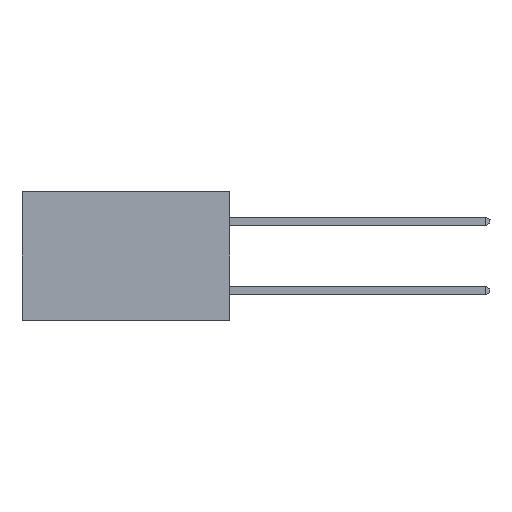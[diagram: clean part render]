
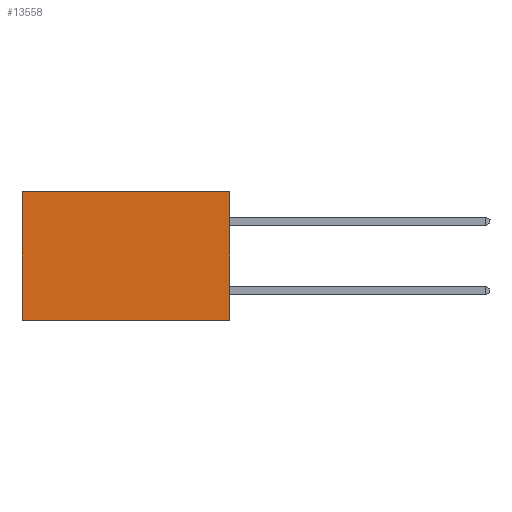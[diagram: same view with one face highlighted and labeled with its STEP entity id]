
A CAD part, left-side view. The second image highlights one B-rep face of the part: STEP entity #13558.
In plain terms, the highlighted planar face has unit normal (-1, 0, 0).
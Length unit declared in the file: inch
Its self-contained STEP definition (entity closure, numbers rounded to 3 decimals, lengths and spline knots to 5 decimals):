
#208 = EDGE_CURVE ( 'NONE', #3559, #17901, #7418, .T. ) ;
#286 = AXIS2_PLACEMENT_3D ( 'NONE', #8222, #3590, #12796 ) ;
#575 = VERTEX_POINT ( 'NONE', #19962 ) ;
#1164 = PLANE ( 'NONE',  #286 ) ;
#3559 = VERTEX_POINT ( 'NONE', #4730 ) ;
#3590 = DIRECTION ( 'NONE',  ( 1., 0., 0. ) ) ;
#4028 = CARTESIAN_POINT ( 'NONE',  ( 0.298, 0., -0.37 ) ) ;
#4073 = EDGE_CURVE ( 'NONE', #17901, #575, #22580, .T. ) ;
#4094 = ORIENTED_EDGE ( 'NONE', *, *, #9278, .T. ) ;
#4730 = CARTESIAN_POINT ( 'NONE',  ( 0.298, 0., 0. ) ) ;
#6565 = LINE ( 'NONE', #22236, #7676 ) ;
#7418 = LINE ( 'NONE', #27569, #8150 ) ;
#7676 = VECTOR ( 'NONE', #22336, 39.37008 ) ;
#8150 = VECTOR ( 'NONE', #11592, 39.37008 ) ;
#8222 = CARTESIAN_POINT ( 'NONE',  ( 0.298, 0., 0. ) ) ;
#8946 = CARTESIAN_POINT ( 'NONE',  ( 0.298, 0.6, 0. ) ) ;
#9278 = EDGE_CURVE ( 'NONE', #11557, #575, #16781, .T. ) ;
#9679 = VECTOR ( 'NONE', #28183, 39.37008 ) ;
#9704 = ORIENTED_EDGE ( 'NONE', *, *, #13098, .T. ) ;
#11557 = VERTEX_POINT ( 'NONE', #8946 ) ;
#11592 = DIRECTION ( 'NONE',  ( 0., 0., -1. ) ) ;
#12796 = DIRECTION ( 'NONE',  ( 0., 0., -1. ) ) ;
#12930 = EDGE_LOOP ( 'NONE', ( #4094, #25171, #25807, #9704 ) ) ;
#13098 = EDGE_CURVE ( 'NONE', #3559, #11557, #6565, .T. ) ;
#13558 = ADVANCED_FACE ( 'NONE', ( #26357 ), #1164, .F. ) ;
#15332 = CARTESIAN_POINT ( 'NONE',  ( 0.298, 0.6, 0. ) ) ;
#16781 = LINE ( 'NONE', #15332, #28743 ) ;
#17901 = VERTEX_POINT ( 'NONE', #4028 ) ;
#18878 = CARTESIAN_POINT ( 'NONE',  ( 0.298, 0., -0.37 ) ) ;
#19962 = CARTESIAN_POINT ( 'NONE',  ( 0.298, 0.6, -0.37 ) ) ;
#22236 = CARTESIAN_POINT ( 'NONE',  ( 0.298, 0., 0. ) ) ;
#22252 = DIRECTION ( 'NONE',  ( 0., 0., -1. ) ) ;
#22336 = DIRECTION ( 'NONE',  ( 0., 1., 0. ) ) ;
#22580 = LINE ( 'NONE', #18878, #9679 ) ;
#25171 = ORIENTED_EDGE ( 'NONE', *, *, #4073, .F. ) ;
#25807 = ORIENTED_EDGE ( 'NONE', *, *, #208, .F. ) ;
#26357 = FACE_OUTER_BOUND ( 'NONE', #12930, .T. ) ;
#27569 = CARTESIAN_POINT ( 'NONE',  ( 0.298, 0., 0. ) ) ;
#28183 = DIRECTION ( 'NONE',  ( 0., 1., 0. ) ) ;
#28743 = VECTOR ( 'NONE', #22252, 39.37008 ) ;
